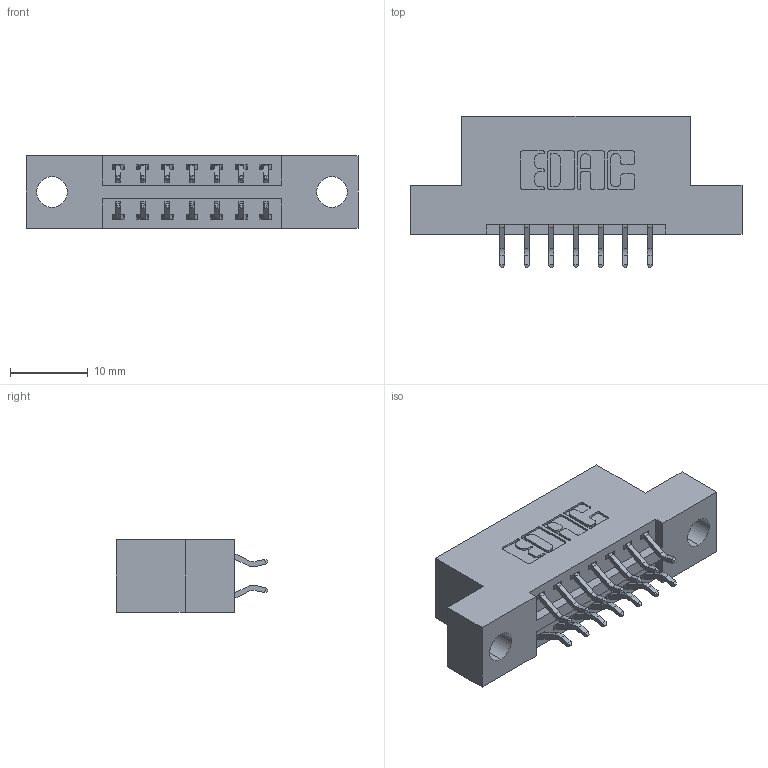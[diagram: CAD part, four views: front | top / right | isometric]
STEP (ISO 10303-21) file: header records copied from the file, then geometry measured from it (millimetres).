
FILE_DESCRIPTION (( 'STEP AP203' ), '1' );
FILE_NAME ('346-014-556-204.STEP', '2022-05-18T14:44:21', ( '' ), ( '' ), 'SwSTEP 2.0', 'SolidWorks 2020', '' );
FILE_SCHEMA (( 'CONFIG_CONTROL_DESIGN' ));
Length unit declared in the file: inch
Products named in the file (3): 345-292-001_556 Tail; 346 Part_Flush Mounting Lugs - 0.156 Dia-TH; 346-014-556-204
Assembly tree (15 placements, depth 2):
  346-014-556-204
    346 Part_Flush Mounting Lugs - 0.156 Dia-TH
    345-292-001_556 Tail  x14
Bounding box: 42.8 x 19.57 x 9.4 mm (x, y, z)
Volume: 3795.1 mm3; surface area: 4501.4 mm2
Topology: 15 solids, 15 shells, 948 faces, 2787 edges, 1838 vertices
Faces by surface type: plane 636, cylinder 312
Entity records: 9919 total; most frequent: CARTESIAN_POINT 1702, ORIENTED_EDGE 1622, DIRECTION 1539, EDGE_CURVE 811, LINE 643, VECTOR 643, VERTEX_POINT 538, AXIS2_PLACEMENT_3D 448
